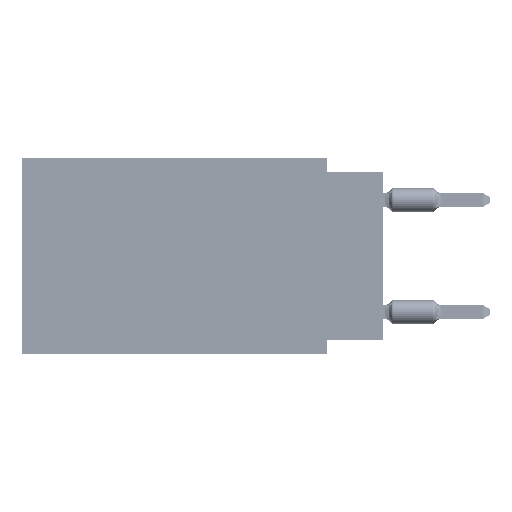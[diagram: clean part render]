
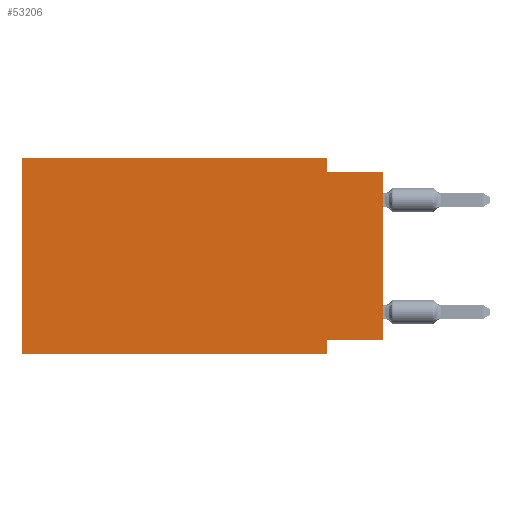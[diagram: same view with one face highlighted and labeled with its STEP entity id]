
A CAD part, left-side view. The second image highlights one B-rep face of the part: STEP entity #53206.
In plain terms, the highlighted planar face has unit normal (-1, 0, 0).
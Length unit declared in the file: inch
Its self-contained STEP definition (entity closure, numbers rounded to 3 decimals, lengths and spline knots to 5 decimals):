
#442 = CARTESIAN_POINT ( 'NONE',  ( 0., 0.645, 0. ) ) ;
#1620 = EDGE_CURVE ( 'NONE', #37656, #34937, #73215, .T. ) ;
#2404 = CARTESIAN_POINT ( 'NONE',  ( 0., 0., 0. ) ) ;
#4757 = VERTEX_POINT ( 'NONE', #8248 ) ;
#7063 = DIRECTION ( 'NONE',  ( 0., -1., 0. ) ) ;
#7073 = LINE ( 'NONE', #48050, #46031 ) ;
#7811 = LINE ( 'NONE', #14682, #58533 ) ;
#8248 = CARTESIAN_POINT ( 'NONE',  ( 0., 0.1, -0.025 ) ) ;
#9999 = PLANE ( 'NONE',  #65070 ) ;
#14682 = CARTESIAN_POINT ( 'NONE',  ( 0., 0.645, -0.35 ) ) ;
#14947 = ORIENTED_EDGE ( 'NONE', *, *, #59961, .F. ) ;
#15248 = VECTOR ( 'NONE', #45596, 39.37008 ) ;
#15364 = CARTESIAN_POINT ( 'NONE',  ( 0., 0.1, 0. ) ) ;
#15811 = ORIENTED_EDGE ( 'NONE', *, *, #54250, .F. ) ;
#17547 = CARTESIAN_POINT ( 'NONE',  ( 0., 0., -0.025 ) ) ;
#17905 = VECTOR ( 'NONE', #50250, 39.37008 ) ;
#18193 = EDGE_CURVE ( 'NONE', #30689, #52444, #7811, .T. ) ;
#18237 = CARTESIAN_POINT ( 'NONE',  ( 0., 0.645, 0. ) ) ;
#18657 = DIRECTION ( 'NONE',  ( 0., 1., 0. ) ) ;
#20223 = ORIENTED_EDGE ( 'NONE', *, *, #18193, .T. ) ;
#23774 = DIRECTION ( 'NONE',  ( 0., -1., 0. ) ) ;
#24409 = VECTOR ( 'NONE', #64001, 39.37008 ) ;
#29115 = LINE ( 'NONE', #53622, #24409 ) ;
#30118 = EDGE_CURVE ( 'NONE', #30689, #30678, #70693, .T. ) ;
#30678 = VERTEX_POINT ( 'NONE', #38885 ) ;
#30689 = VERTEX_POINT ( 'NONE', #62266 ) ;
#32964 = EDGE_CURVE ( 'NONE', #30678, #43734, #52897, .T. ) ;
#33877 = ORIENTED_EDGE ( 'NONE', *, *, #65535, .F. ) ;
#34937 = VERTEX_POINT ( 'NONE', #17547 ) ;
#35073 = VECTOR ( 'NONE', #23774, 39.37008 ) ;
#37656 = VERTEX_POINT ( 'NONE', #63439 ) ;
#38218 = CARTESIAN_POINT ( 'NONE',  ( 0., 0.1, -0.35 ) ) ;
#38690 = ORIENTED_EDGE ( 'NONE', *, *, #1620, .T. ) ;
#38885 = CARTESIAN_POINT ( 'NONE',  ( 0., 0.645, 0. ) ) ;
#41137 = ORIENTED_EDGE ( 'NONE', *, *, #32964, .F. ) ;
#43014 = DIRECTION ( 'NONE',  ( 0., -1., 0. ) ) ;
#43090 = EDGE_CURVE ( 'NONE', #4757, #34937, #65283, .T. ) ;
#43193 = VECTOR ( 'NONE', #18657, 39.37008 ) ;
#43734 = VERTEX_POINT ( 'NONE', #15364 ) ;
#44075 = DIRECTION ( 'NONE',  ( 0., 0., -1. ) ) ;
#45503 = ORIENTED_EDGE ( 'NONE', *, *, #43090, .F. ) ;
#45596 = DIRECTION ( 'NONE',  ( 0., 0., 1. ) ) ;
#46031 = VECTOR ( 'NONE', #66038, 39.37008 ) ;
#47182 = VECTOR ( 'NONE', #7063, 39.37008 ) ;
#47750 = CARTESIAN_POINT ( 'NONE',  ( 0., 0., -0.325 ) ) ;
#48050 = CARTESIAN_POINT ( 'NONE',  ( 0., 0.1, -0.35 ) ) ;
#48897 = LINE ( 'NONE', #47750, #43193 ) ;
#50250 = DIRECTION ( 'NONE',  ( 0., 0., 1. ) ) ;
#50974 = FACE_OUTER_BOUND ( 'NONE', #53871, .T. ) ;
#52444 = VERTEX_POINT ( 'NONE', #38218 ) ;
#52897 = LINE ( 'NONE', #442, #35073 ) ;
#53206 = ADVANCED_FACE ( 'NONE', ( #50974 ), #9999, .F. ) ;
#53622 = CARTESIAN_POINT ( 'NONE',  ( 0., 0.1, 0. ) ) ;
#53871 = EDGE_LOOP ( 'NONE', ( #38690, #45503, #33877, #41137, #72434, #20223, #14947, #15811 ) ) ;
#54250 = EDGE_CURVE ( 'NONE', #37656, #56431, #48897, .T. ) ;
#56431 = VERTEX_POINT ( 'NONE', #68609 ) ;
#58533 = VECTOR ( 'NONE', #43014, 39.37008 ) ;
#59510 = CARTESIAN_POINT ( 'NONE',  ( 0., 0., -0.025 ) ) ;
#59961 = EDGE_CURVE ( 'NONE', #56431, #52444, #7073, .T. ) ;
#62266 = CARTESIAN_POINT ( 'NONE',  ( 0., 0.645, -0.35 ) ) ;
#63439 = CARTESIAN_POINT ( 'NONE',  ( 0., 0., -0.325 ) ) ;
#64001 = DIRECTION ( 'NONE',  ( 0., 0., -1. ) ) ;
#65070 = AXIS2_PLACEMENT_3D ( 'NONE', #68594, #75085, #44075 ) ;
#65283 = LINE ( 'NONE', #59510, #47182 ) ;
#65535 = EDGE_CURVE ( 'NONE', #43734, #4757, #29115, .T. ) ;
#66038 = DIRECTION ( 'NONE',  ( 0., 0., -1. ) ) ;
#68594 = CARTESIAN_POINT ( 'NONE',  ( 0., 0.645, 0. ) ) ;
#68609 = CARTESIAN_POINT ( 'NONE',  ( 0., 0.1, -0.325 ) ) ;
#70693 = LINE ( 'NONE', #18237, #15248 ) ;
#72434 = ORIENTED_EDGE ( 'NONE', *, *, #30118, .F. ) ;
#73215 = LINE ( 'NONE', #2404, #17905 ) ;
#75085 = DIRECTION ( 'NONE',  ( 1., 0., 0. ) ) ;
